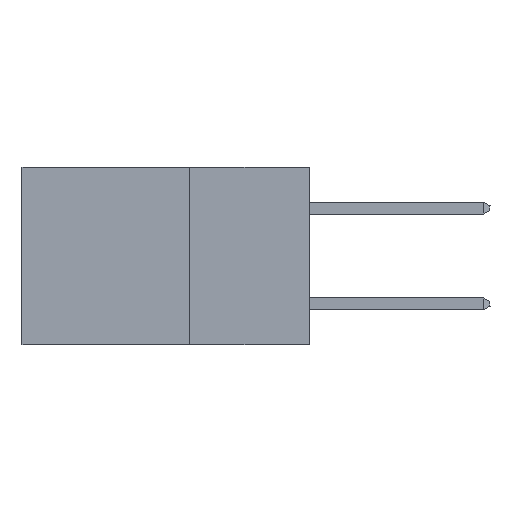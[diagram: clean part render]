
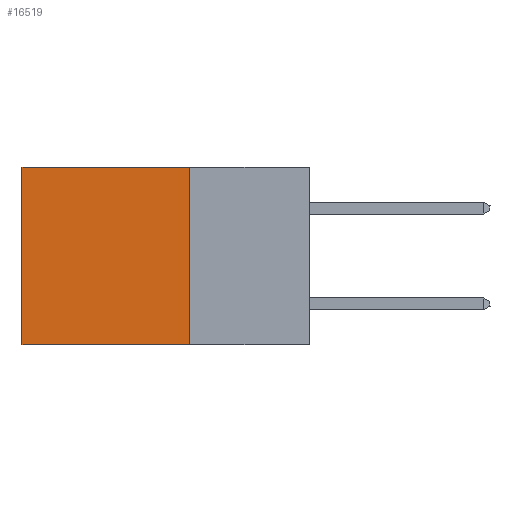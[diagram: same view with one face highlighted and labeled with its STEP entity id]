
A CAD part, left-side view. The second image highlights one B-rep face of the part: STEP entity #16519.
In plain terms, the highlighted planar face has unit normal (-1, 0, 0).
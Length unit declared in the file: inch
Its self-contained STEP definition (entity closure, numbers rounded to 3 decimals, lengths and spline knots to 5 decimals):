
#489 = VERTEX_POINT ( 'NONE', #26708 ) ;
#1313 = LINE ( 'NONE', #4213, #6777 ) ;
#1872 = ORIENTED_EDGE ( 'NONE', *, *, #10114, .T. ) ;
#2457 = ORIENTED_EDGE ( 'NONE', *, *, #27461, .T. ) ;
#3693 = EDGE_CURVE ( 'NONE', #489, #27149, #6912, .T. ) ;
#4213 = CARTESIAN_POINT ( 'NONE',  ( 0.2875, 0.25, -0.37 ) ) ;
#4412 = VERTEX_POINT ( 'NONE', #19193 ) ;
#4643 = AXIS2_PLACEMENT_3D ( 'NONE', #23286, #4996, #21135 ) ;
#4996 = DIRECTION ( 'NONE',  ( 1., 0., 0. ) ) ;
#6290 = VERTEX_POINT ( 'NONE', #14153 ) ;
#6433 = CARTESIAN_POINT ( 'NONE',  ( 0.2875, 0.6, 0. ) ) ;
#6777 = VECTOR ( 'NONE', #18137, 39.37008 ) ;
#6912 = LINE ( 'NONE', #7492, #25162 ) ;
#7063 = DIRECTION ( 'NONE',  ( 0., 0., -1. ) ) ;
#7492 = CARTESIAN_POINT ( 'NONE',  ( 0.2875, 0.25, 0. ) ) ;
#9179 = ORIENTED_EDGE ( 'NONE', *, *, #25989, .F. ) ;
#10114 = EDGE_CURVE ( 'NONE', #489, #6290, #14607, .T. ) ;
#14153 = CARTESIAN_POINT ( 'NONE',  ( 0.2875, 0.6, 0. ) ) ;
#14607 = LINE ( 'NONE', #28768, #20625 ) ;
#15425 = DIRECTION ( 'NONE',  ( 0., 1., 0. ) ) ;
#16519 = ADVANCED_FACE ( 'NONE', ( #23809 ), #18871, .F. ) ;
#17153 = EDGE_LOOP ( 'NONE', ( #2457, #9179, #28201, #1872 ) ) ;
#18137 = DIRECTION ( 'NONE',  ( 0., 1., 0. ) ) ;
#18656 = LINE ( 'NONE', #6433, #24592 ) ;
#18871 = PLANE ( 'NONE',  #4643 ) ;
#19193 = CARTESIAN_POINT ( 'NONE',  ( 0.2875, 0.6, -0.37 ) ) ;
#20625 = VECTOR ( 'NONE', #15425, 39.37008 ) ;
#21135 = DIRECTION ( 'NONE',  ( 0., 0., -1. ) ) ;
#23286 = CARTESIAN_POINT ( 'NONE',  ( 0.2875, 0.25, 0. ) ) ;
#23809 = FACE_OUTER_BOUND ( 'NONE', #17153, .T. ) ;
#24592 = VECTOR ( 'NONE', #7063, 39.37008 ) ;
#25162 = VECTOR ( 'NONE', #25736, 39.37008 ) ;
#25736 = DIRECTION ( 'NONE',  ( 0., 0., -1. ) ) ;
#25989 = EDGE_CURVE ( 'NONE', #27149, #4412, #1313, .T. ) ;
#26407 = CARTESIAN_POINT ( 'NONE',  ( 0.2875, 0.25, -0.37 ) ) ;
#26708 = CARTESIAN_POINT ( 'NONE',  ( 0.2875, 0.25, 0. ) ) ;
#27149 = VERTEX_POINT ( 'NONE', #26407 ) ;
#27461 = EDGE_CURVE ( 'NONE', #6290, #4412, #18656, .T. ) ;
#28201 = ORIENTED_EDGE ( 'NONE', *, *, #3693, .F. ) ;
#28768 = CARTESIAN_POINT ( 'NONE',  ( 0.2875, 0.25, 0. ) ) ;
